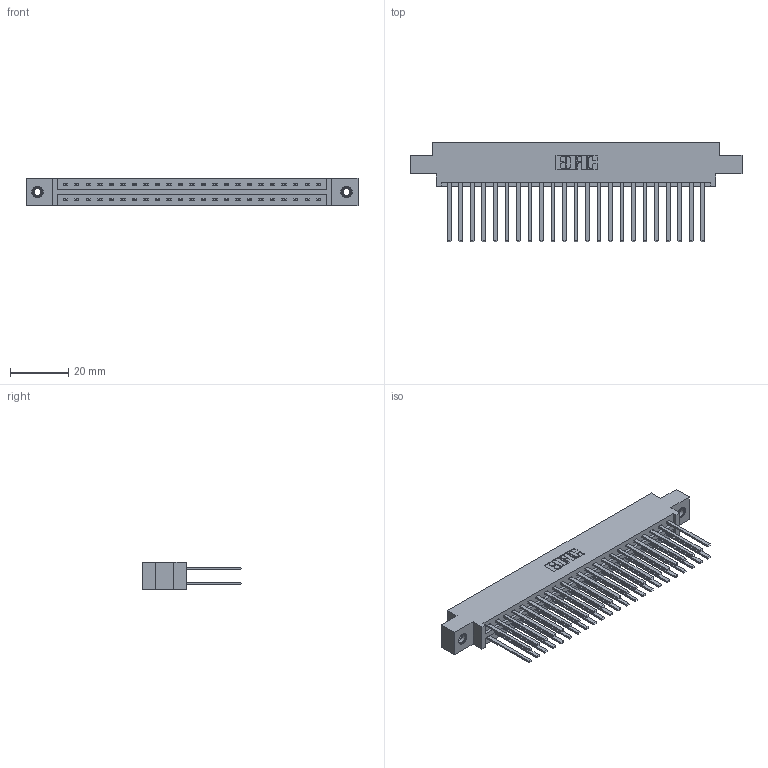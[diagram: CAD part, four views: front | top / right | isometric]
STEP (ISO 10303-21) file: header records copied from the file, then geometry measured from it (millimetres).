
FILE_DESCRIPTION (( 'STEP AP203' ), '1' );
FILE_NAME ('337-046-544-808.STEP', '2019-10-11T14:41:52', ( '' ), ( '' ), 'SwSTEP 2.0', 'SolidWorks 2016', '' );
FILE_SCHEMA (( 'CONFIG_CONTROL_DESIGN' ));
Length unit declared in the file: inch
Products named in the file (4): 345-250-001_345-250-003-102; 345-292-001_345-293-144; 337-046-544-808; 337 Part_0.170 Offset - 0.156 Dia-TI
Assembly tree (49 placements, depth 2):
  337-046-544-808
    337 Part_0.170 Offset - 0.156 Dia-TI
    345-292-001_345-293-144  x46
    345-250-001_345-250-003-102  x2
Bounding box: 114.15 x 34.3 x 9.4 mm (x, y, z)
Volume: 12297.7 mm3; surface area: 15956.3 mm2
Topology: 49 solids, 49 shells, 2386 faces, 7037 edges, 4622 vertices
Faces by surface type: plane 1670, cylinder 700, cone 12, torus 4
Entity records: 21424 total; most frequent: CARTESIAN_POINT 3605, ORIENTED_EDGE 3534, DIRECTION 3129, EDGE_CURVE 1767, VECTOR 1623, LINE 1623, VERTEX_POINT 1172, AXIS2_PLACEMENT_3D 753
